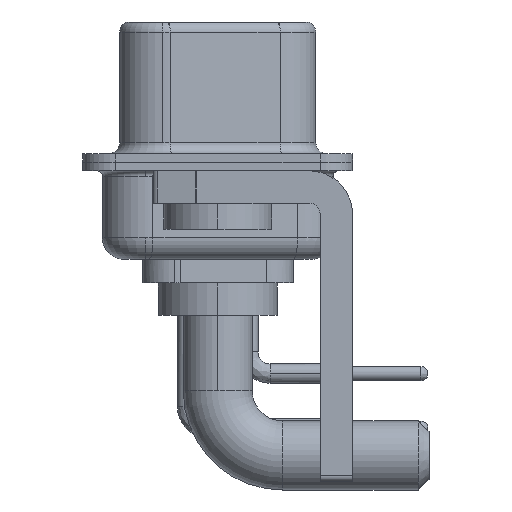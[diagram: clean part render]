
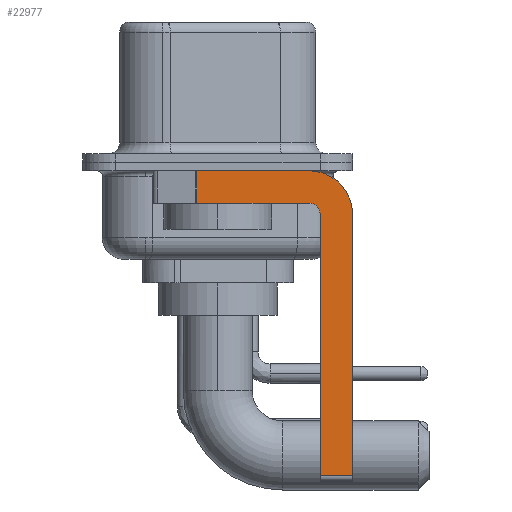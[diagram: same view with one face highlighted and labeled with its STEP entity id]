
A CAD part, left-side view. The second image highlights one B-rep face of the part: STEP entity #22977.
In plain terms, the highlighted planar face has unit normal (-1, 0, 0).
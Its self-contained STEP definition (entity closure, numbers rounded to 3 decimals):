
#91 = EDGE_LOOP ( 'NONE', ( #22082, #4441, #10568, #16964, #16710, #11703, #26592, #13855 ) ) ;
#581 = LINE ( 'NONE', #8783, #2851 ) ;
#728 = VECTOR ( 'NONE', #13705, 1000. ) ;
#949 = EDGE_CURVE ( 'NONE', #25883, #24816, #5562, .T. ) ;
#1201 = VERTEX_POINT ( 'NONE', #13218 ) ;
#1659 = CARTESIAN_POINT ( 'NONE',  ( -2.9, 0.978, -0.4 ) ) ;
#1699 = VERTEX_POINT ( 'NONE', #14979 ) ;
#2842 = DIRECTION ( 'NONE',  ( 1., 0., 0. ) ) ;
#2851 = VECTOR ( 'NONE', #17004, 1000. ) ;
#3259 = LINE ( 'NONE', #19384, #4695 ) ;
#3719 = CARTESIAN_POINT ( 'NONE',  ( -2.9, -6.25, -14.55 ) ) ;
#3726 = CARTESIAN_POINT ( 'NONE',  ( -2.9, 0.978, -1.9 ) ) ;
#4441 = ORIENTED_EDGE ( 'NONE', *, *, #22322, .T. ) ;
#4695 = VECTOR ( 'NONE', #23552, 1000. ) ;
#4760 = CARTESIAN_POINT ( 'NONE',  ( -2.9, -4.25, -2.4 ) ) ;
#5017 = VERTEX_POINT ( 'NONE', #1659 ) ;
#5531 = CARTESIAN_POINT ( 'NONE',  ( -2.9, -4.25, -2.4 ) ) ;
#5562 = LINE ( 'NONE', #24109, #12969 ) ;
#5864 = AXIS2_PLACEMENT_3D ( 'NONE', #20868, #2842, #21398 ) ;
#6384 = DIRECTION ( 'NONE',  ( -1., 0., 0. ) ) ;
#6734 = PLANE ( 'NONE',  #5864 ) ;
#7273 = VERTEX_POINT ( 'NONE', #3726 ) ;
#7515 = CIRCLE ( 'NONE', #22127, 0.5 ) ;
#8365 = VERTEX_POINT ( 'NONE', #11158 ) ;
#8783 = CARTESIAN_POINT ( 'NONE',  ( -2.9, 3., -0.4 ) ) ;
#9218 = LINE ( 'NONE', #23057, #9936 ) ;
#9593 = VECTOR ( 'NONE', #26252, 1000. ) ;
#9936 = VECTOR ( 'NONE', #13127, 1000. ) ;
#10568 = ORIENTED_EDGE ( 'NONE', *, *, #25666, .F. ) ;
#11158 = CARTESIAN_POINT ( 'NONE',  ( -2.9, -4.25, -0.4 ) ) ;
#11703 = ORIENTED_EDGE ( 'NONE', *, *, #17826, .T. ) ;
#11743 = EDGE_CURVE ( 'NONE', #8365, #25883, #25920, .T. ) ;
#12867 = EDGE_CURVE ( 'NONE', #1201, #15224, #7515, .T. ) ;
#12969 = VECTOR ( 'NONE', #13780, 1000. ) ;
#13127 = DIRECTION ( 'NONE',  ( 0., 0., 1. ) ) ;
#13218 = CARTESIAN_POINT ( 'NONE',  ( -2.9, -4.75, -2.4 ) ) ;
#13705 = DIRECTION ( 'NONE',  ( 0., 0., -1. ) ) ;
#13780 = DIRECTION ( 'NONE',  ( 0., 0., -1. ) ) ;
#13855 = ORIENTED_EDGE ( 'NONE', *, *, #11743, .F. ) ;
#13901 = CARTESIAN_POINT ( 'NONE',  ( -2.9, -4.25, -1.9 ) ) ;
#14653 = EDGE_CURVE ( 'NONE', #1699, #1201, #9218, .T. ) ;
#14979 = CARTESIAN_POINT ( 'NONE',  ( -2.9, -4.75, -14.55 ) ) ;
#15224 = VERTEX_POINT ( 'NONE', #13901 ) ;
#16056 = CARTESIAN_POINT ( 'NONE',  ( -2.9, -4.25, -14.55 ) ) ;
#16149 = CARTESIAN_POINT ( 'NONE',  ( -2.9, -6.25, -2.4 ) ) ;
#16710 = ORIENTED_EDGE ( 'NONE', *, *, #14653, .F. ) ;
#16878 = DIRECTION ( 'NONE',  ( 0., 0., 1. ) ) ;
#16964 = ORIENTED_EDGE ( 'NONE', *, *, #12867, .F. ) ;
#17004 = DIRECTION ( 'NONE',  ( 0., -1., 0. ) ) ;
#17826 = EDGE_CURVE ( 'NONE', #1699, #24816, #21961, .T. ) ;
#19127 = FACE_OUTER_BOUND ( 'NONE', #91, .T. ) ;
#19384 = CARTESIAN_POINT ( 'NONE',  ( -2.9, -4.25, -1.9 ) ) ;
#19739 = CARTESIAN_POINT ( 'NONE',  ( -2.9, 0.978, -1.9 ) ) ;
#19784 = DIRECTION ( 'NONE',  ( 0., 0., -1. ) ) ;
#20868 = CARTESIAN_POINT ( 'NONE',  ( -2.9, -4.25, -2.4 ) ) ;
#21398 = DIRECTION ( 'NONE',  ( 0., 0., -1. ) ) ;
#21961 = LINE ( 'NONE', #16056, #9593 ) ;
#22082 = ORIENTED_EDGE ( 'NONE', *, *, #22652, .F. ) ;
#22127 = AXIS2_PLACEMENT_3D ( 'NONE', #4760, #6384, #16878 ) ;
#22322 = EDGE_CURVE ( 'NONE', #5017, #7273, #23904, .T. ) ;
#22652 = EDGE_CURVE ( 'NONE', #5017, #8365, #581, .T. ) ;
#22977 = ADVANCED_FACE ( 'NONE', ( #19127 ), #6734, .F. ) ;
#23057 = CARTESIAN_POINT ( 'NONE',  ( -2.9, -4.75, -14.8 ) ) ;
#23552 = DIRECTION ( 'NONE',  ( 0., 1., 0. ) ) ;
#23904 = LINE ( 'NONE', #19739, #728 ) ;
#24109 = CARTESIAN_POINT ( 'NONE',  ( -2.9, -6.25, -2.4 ) ) ;
#24816 = VERTEX_POINT ( 'NONE', #3719 ) ;
#25055 = AXIS2_PLACEMENT_3D ( 'NONE', #5531, #25822, #19784 ) ;
#25666 = EDGE_CURVE ( 'NONE', #15224, #7273, #3259, .T. ) ;
#25822 = DIRECTION ( 'NONE',  ( 1., 0., 0. ) ) ;
#25883 = VERTEX_POINT ( 'NONE', #16149 ) ;
#25920 = CIRCLE ( 'NONE', #25055, 2. ) ;
#26252 = DIRECTION ( 'NONE',  ( 0., -1., 0. ) ) ;
#26592 = ORIENTED_EDGE ( 'NONE', *, *, #949, .F. ) ;
